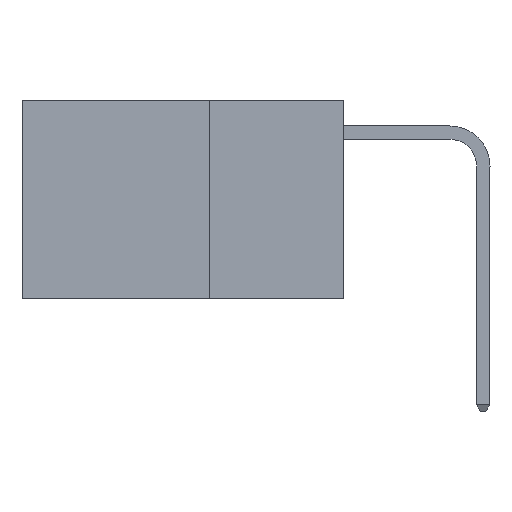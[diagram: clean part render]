
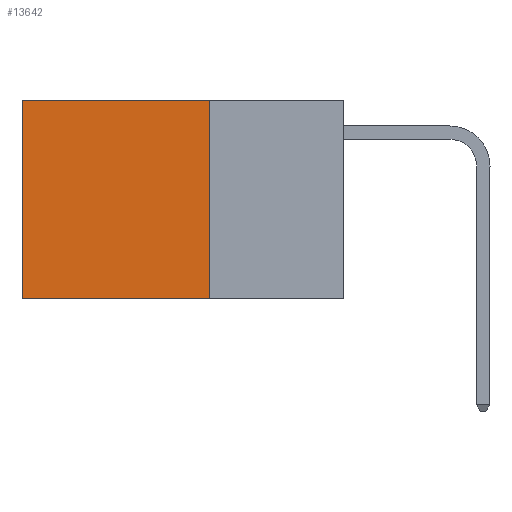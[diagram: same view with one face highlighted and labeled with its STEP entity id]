
A CAD part, left-side view. The second image highlights one B-rep face of the part: STEP entity #13642.
In plain terms, the highlighted planar face has unit normal (-1, 0, 0).
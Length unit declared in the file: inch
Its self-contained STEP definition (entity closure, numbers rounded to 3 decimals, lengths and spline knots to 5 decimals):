
#639 = PLANE ( 'NONE',  #14148 ) ;
#916 = ORIENTED_EDGE ( 'NONE', *, *, #5436, .T. ) ;
#1077 = EDGE_CURVE ( 'NONE', #9353, #2472, #15160, .T. ) ;
#1484 = ORIENTED_EDGE ( 'NONE', *, *, #1928, .F. ) ;
#1921 = DIRECTION ( 'NONE',  ( 1., 0., 0. ) ) ;
#1928 = EDGE_CURVE ( 'NONE', #2472, #12340, #4022, .T. ) ;
#2169 = CARTESIAN_POINT ( 'NONE',  ( 0.2625, 0.6, 0. ) ) ;
#2472 = VERTEX_POINT ( 'NONE', #8395 ) ;
#2957 = ORIENTED_EDGE ( 'NONE', *, *, #1077, .F. ) ;
#3299 = DIRECTION ( 'NONE',  ( 0., 1., 0. ) ) ;
#3450 = DIRECTION ( 'NONE',  ( 0., 0., -1. ) ) ;
#4022 = LINE ( 'NONE', #10652, #14276 ) ;
#4353 = FACE_OUTER_BOUND ( 'NONE', #4417, .T. ) ;
#4417 = EDGE_LOOP ( 'NONE', ( #916, #1484, #2957, #6319 ) ) ;
#4623 = CARTESIAN_POINT ( 'NONE',  ( 0.2625, 0.6, 0. ) ) ;
#5436 = EDGE_CURVE ( 'NONE', #13788, #12340, #7068, .T. ) ;
#6319 = ORIENTED_EDGE ( 'NONE', *, *, #9481, .T. ) ;
#6336 = VECTOR ( 'NONE', #3450, 39.37008 ) ;
#6692 = CARTESIAN_POINT ( 'NONE',  ( 0.2625, 0.25, 0. ) ) ;
#7068 = LINE ( 'NONE', #4623, #6336 ) ;
#7920 = CARTESIAN_POINT ( 'NONE',  ( 0.2625, 0.6, -0.37 ) ) ;
#8395 = CARTESIAN_POINT ( 'NONE',  ( 0.2625, 0.25, -0.37 ) ) ;
#9151 = CARTESIAN_POINT ( 'NONE',  ( 0.2625, 0.25, 0. ) ) ;
#9199 = DIRECTION ( 'NONE',  ( 0., 0., -1. ) ) ;
#9310 = VECTOR ( 'NONE', #9199, 39.37008 ) ;
#9353 = VERTEX_POINT ( 'NONE', #6692 ) ;
#9481 = EDGE_CURVE ( 'NONE', #9353, #13788, #12385, .T. ) ;
#10365 = DIRECTION ( 'NONE',  ( 0., 0., -1. ) ) ;
#10418 = CARTESIAN_POINT ( 'NONE',  ( 0.2625, 0.25, 0. ) ) ;
#10652 = CARTESIAN_POINT ( 'NONE',  ( 0.2625, 0.25, -0.37 ) ) ;
#11732 = CARTESIAN_POINT ( 'NONE',  ( 0.2625, 0.25, 0. ) ) ;
#12340 = VERTEX_POINT ( 'NONE', #7920 ) ;
#12385 = LINE ( 'NONE', #11732, #15035 ) ;
#13025 = DIRECTION ( 'NONE',  ( 0., 1., 0. ) ) ;
#13642 = ADVANCED_FACE ( 'NONE', ( #4353 ), #639, .F. ) ;
#13788 = VERTEX_POINT ( 'NONE', #2169 ) ;
#14148 = AXIS2_PLACEMENT_3D ( 'NONE', #9151, #1921, #10365 ) ;
#14276 = VECTOR ( 'NONE', #13025, 39.37008 ) ;
#15035 = VECTOR ( 'NONE', #3299, 39.37008 ) ;
#15160 = LINE ( 'NONE', #10418, #9310 ) ;
